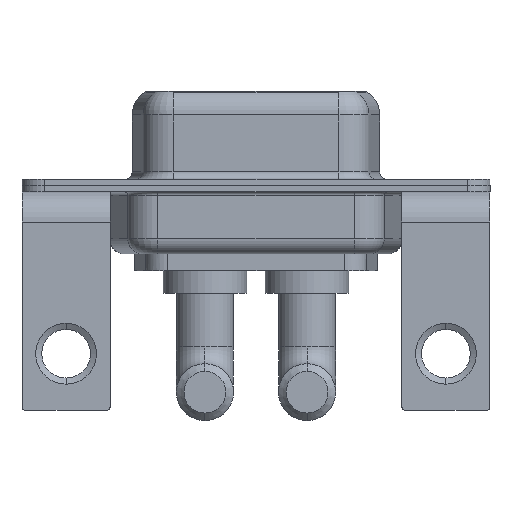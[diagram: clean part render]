
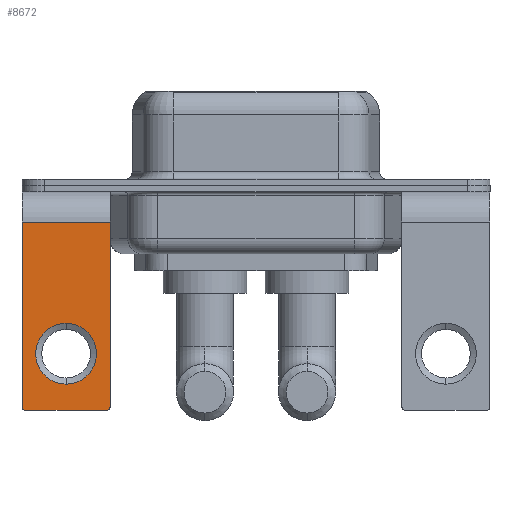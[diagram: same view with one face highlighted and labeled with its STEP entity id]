
A CAD part, front view. The second image highlights one B-rep face of the part: STEP entity #8672.
In plain terms, the highlighted planar face has unit normal (0, -1, 0).
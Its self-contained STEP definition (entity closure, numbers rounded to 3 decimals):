
#105 = DIRECTION ( 'NONE',  ( -1., 0., 0. ) ) ;
#148 = DIRECTION ( 'NONE',  ( 0., 0., -1. ) ) ;
#643 = EDGE_CURVE ( 'NONE', #1487, #11516, #5243, .T. ) ;
#713 = ORIENTED_EDGE ( 'NONE', *, *, #5808, .F. ) ;
#794 = ORIENTED_EDGE ( 'NONE', *, *, #643, .T. ) ;
#973 = ORIENTED_EDGE ( 'NONE', *, *, #4896, .F. ) ;
#982 = CARTESIAN_POINT ( 'NONE',  ( 2.65, -6.25, -14.8 ) ) ;
#1236 = VERTEX_POINT ( 'NONE', #10047 ) ;
#1313 = CARTESIAN_POINT ( 'NONE',  ( -2.9, -6.25, -14.55 ) ) ;
#1487 = VERTEX_POINT ( 'NONE', #1313 ) ;
#2068 = DIRECTION ( 'NONE',  ( 0., 0., 1. ) ) ;
#2512 = CARTESIAN_POINT ( 'NONE',  ( 0., -6.25, -13.07 ) ) ;
#2804 = VECTOR ( 'NONE', #3114, 1000. ) ;
#2917 = DIRECTION ( 'NONE',  ( 0., 0., 1. ) ) ;
#3114 = DIRECTION ( 'NONE',  ( -1., 0., 0. ) ) ;
#3118 = CARTESIAN_POINT ( 'NONE',  ( 2.9, -6.25, -2.4 ) ) ;
#3510 = CARTESIAN_POINT ( 'NONE',  ( 0., -6.25, -9.07 ) ) ;
#3703 = AXIS2_PLACEMENT_3D ( 'NONE', #9351, #11438, #6528 ) ;
#3803 = ORIENTED_EDGE ( 'NONE', *, *, #10380, .T. ) ;
#3907 = AXIS2_PLACEMENT_3D ( 'NONE', #3118, #7960, #2068 ) ;
#4470 = VECTOR ( 'NONE', #148, 1000. ) ;
#4647 = CIRCLE ( 'NONE', #11741, 2. ) ;
#4736 = EDGE_CURVE ( 'NONE', #5898, #9366, #5076, .T. ) ;
#4742 = CARTESIAN_POINT ( 'NONE',  ( 0., -6.25, -11.07 ) ) ;
#4867 = DIRECTION ( 'NONE',  ( 0., 0., 1. ) ) ;
#4896 = EDGE_CURVE ( 'NONE', #1236, #8558, #10034, .T. ) ;
#4941 = LINE ( 'NONE', #8075, #6616 ) ;
#5076 = CIRCLE ( 'NONE', #6341, 2. ) ;
#5208 = PLANE ( 'NONE',  #3907 ) ;
#5243 = CIRCLE ( 'NONE', #6071, 0.25 ) ;
#5358 = EDGE_LOOP ( 'NONE', ( #3803, #10538 ) ) ;
#5602 = CARTESIAN_POINT ( 'NONE',  ( 0., -6.25, -11.07 ) ) ;
#5808 = EDGE_CURVE ( 'NONE', #12638, #11516, #8093, .T. ) ;
#5898 = VERTEX_POINT ( 'NONE', #3510 ) ;
#6024 = VECTOR ( 'NONE', #105, 1000. ) ;
#6071 = AXIS2_PLACEMENT_3D ( 'NONE', #10719, #8821, #12740 ) ;
#6341 = AXIS2_PLACEMENT_3D ( 'NONE', #4742, #8791, #4867 ) ;
#6528 = DIRECTION ( 'NONE',  ( 0., 0., 1. ) ) ;
#6616 = VECTOR ( 'NONE', #10831, 1000. ) ;
#6774 = DIRECTION ( 'NONE',  ( 0., 1., 0. ) ) ;
#7061 = CARTESIAN_POINT ( 'NONE',  ( -2.65, -6.25, -14.8 ) ) ;
#7250 = CIRCLE ( 'NONE', #3703, 0.25 ) ;
#7849 = EDGE_CURVE ( 'NONE', #10351, #1487, #4941, .T. ) ;
#7960 = DIRECTION ( 'NONE',  ( 0., 1., 0. ) ) ;
#8075 = CARTESIAN_POINT ( 'NONE',  ( -2.9, -6.25, -2.4 ) ) ;
#8093 = LINE ( 'NONE', #10384, #2804 ) ;
#8353 = EDGE_CURVE ( 'NONE', #12638, #8558, #7250, .T. ) ;
#8558 = VERTEX_POINT ( 'NONE', #12737 ) ;
#8559 = ORIENTED_EDGE ( 'NONE', *, *, #8739, .T. ) ;
#8672 = ADVANCED_FACE ( 'NONE', ( #12801, #11826 ), #5208, .F. ) ;
#8739 = EDGE_CURVE ( 'NONE', #1236, #10351, #9196, .T. ) ;
#8791 = DIRECTION ( 'NONE',  ( 0., 1., 0. ) ) ;
#8821 = DIRECTION ( 'NONE',  ( 0., -1., 0. ) ) ;
#8949 = CARTESIAN_POINT ( 'NONE',  ( 2.9, -6.25, -2.4 ) ) ;
#9048 = CARTESIAN_POINT ( 'NONE',  ( 2.9, -6.25, -2.4 ) ) ;
#9196 = LINE ( 'NONE', #8949, #6024 ) ;
#9351 = CARTESIAN_POINT ( 'NONE',  ( 2.65, -6.25, -14.55 ) ) ;
#9366 = VERTEX_POINT ( 'NONE', #2512 ) ;
#9900 = ORIENTED_EDGE ( 'NONE', *, *, #7849, .T. ) ;
#10034 = LINE ( 'NONE', #9048, #4470 ) ;
#10047 = CARTESIAN_POINT ( 'NONE',  ( 2.9, -6.25, -2.4 ) ) ;
#10351 = VERTEX_POINT ( 'NONE', #12158 ) ;
#10380 = EDGE_CURVE ( 'NONE', #9366, #5898, #4647, .T. ) ;
#10384 = CARTESIAN_POINT ( 'NONE',  ( 2.9, -6.25, -14.8 ) ) ;
#10538 = ORIENTED_EDGE ( 'NONE', *, *, #4736, .T. ) ;
#10719 = CARTESIAN_POINT ( 'NONE',  ( -2.65, -6.25, -14.55 ) ) ;
#10831 = DIRECTION ( 'NONE',  ( 0., 0., -1. ) ) ;
#11181 = ORIENTED_EDGE ( 'NONE', *, *, #8353, .T. ) ;
#11438 = DIRECTION ( 'NONE',  ( 0., -1., 0. ) ) ;
#11516 = VERTEX_POINT ( 'NONE', #7061 ) ;
#11741 = AXIS2_PLACEMENT_3D ( 'NONE', #5602, #6774, #2917 ) ;
#11826 = FACE_OUTER_BOUND ( 'NONE', #12942, .T. ) ;
#12158 = CARTESIAN_POINT ( 'NONE',  ( -2.9, -6.25, -2.4 ) ) ;
#12638 = VERTEX_POINT ( 'NONE', #982 ) ;
#12737 = CARTESIAN_POINT ( 'NONE',  ( 2.9, -6.25, -14.55 ) ) ;
#12740 = DIRECTION ( 'NONE',  ( 0., 0., 1. ) ) ;
#12801 = FACE_BOUND ( 'NONE', #5358, .T. ) ;
#12942 = EDGE_LOOP ( 'NONE', ( #9900, #794, #713, #11181, #973, #8559 ) ) ;
